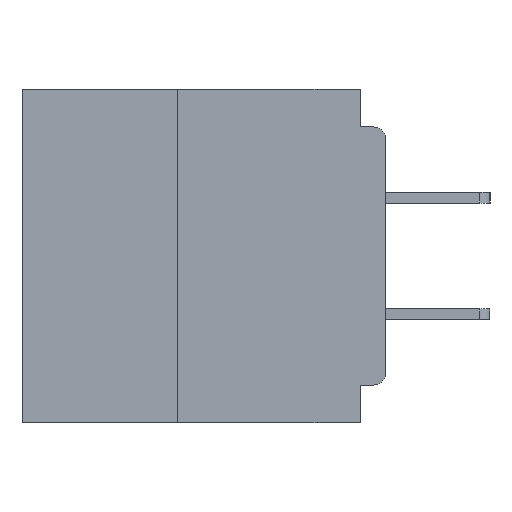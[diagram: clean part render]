
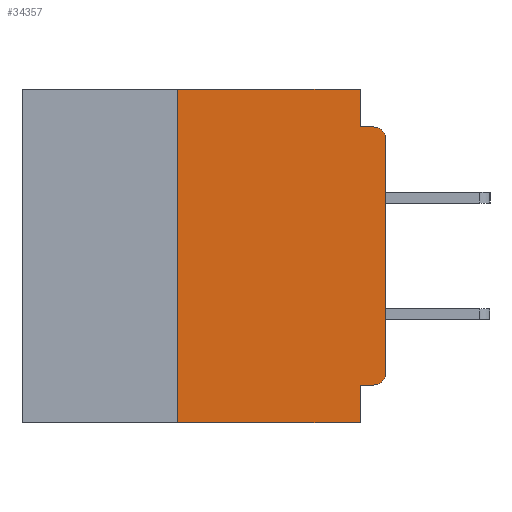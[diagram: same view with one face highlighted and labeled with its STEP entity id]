
A CAD part, left-side view. The second image highlights one B-rep face of the part: STEP entity #34357.
In plain terms, the highlighted planar face has unit normal (-1, 0, 0).
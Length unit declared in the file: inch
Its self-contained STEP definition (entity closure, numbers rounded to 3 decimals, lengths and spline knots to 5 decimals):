
#876 = AXIS2_PLACEMENT_3D ( 'NONE', #6348, #29457, #9717 ) ;
#1422 = DIRECTION ( 'NONE',  ( 1., 0., 0. ) ) ;
#1645 = CARTESIAN_POINT ( 'NONE',  ( 0., 0., -0.06 ) ) ;
#1681 = ORIENTED_EDGE ( 'NONE', *, *, #37611, .T. ) ;
#2135 = VECTOR ( 'NONE', #24964, 39.37008 ) ;
#2602 = LINE ( 'NONE', #12589, #36642 ) ;
#2660 = CARTESIAN_POINT ( 'NONE',  ( 0., 0.25, 0. ) ) ;
#3828 = EDGE_LOOP ( 'NONE', ( #1681, #27173, #12456, #31280, #8950, #22543, #33242, #8551, #8902, #25449 ) ) ;
#4200 = DIRECTION ( 'NONE',  ( 0., 0., -1. ) ) ;
#5131 = CARTESIAN_POINT ( 'NONE',  ( 0., 0.031, -0.4 ) ) ;
#6348 = CARTESIAN_POINT ( 'NONE',  ( 0., 0.015, -0.34 ) ) ;
#7102 = VERTEX_POINT ( 'NONE', #30619 ) ;
#7953 = EDGE_CURVE ( 'NONE', #16757, #12683, #25934, .T. ) ;
#8014 = CARTESIAN_POINT ( 'NONE',  ( 0., 0.437, 0. ) ) ;
#8551 = ORIENTED_EDGE ( 'NONE', *, *, #33032, .F. ) ;
#8730 = DIRECTION ( 'NONE',  ( -1., 0., 0. ) ) ;
#8902 = ORIENTED_EDGE ( 'NONE', *, *, #31078, .F. ) ;
#8950 = ORIENTED_EDGE ( 'NONE', *, *, #7953, .F. ) ;
#9042 = LINE ( 'NONE', #31678, #41821 ) ;
#9165 = FACE_OUTER_BOUND ( 'NONE', #3828, .T. ) ;
#9479 = EDGE_CURVE ( 'NONE', #12995, #27220, #18649, .T. ) ;
#9717 = DIRECTION ( 'NONE',  ( 0., 0., -1. ) ) ;
#9945 = VERTEX_POINT ( 'NONE', #10991 ) ;
#10199 = CIRCLE ( 'NONE', #24313, 0.015 ) ;
#10349 = VECTOR ( 'NONE', #4200, 39.37008 ) ;
#10695 = EDGE_CURVE ( 'NONE', #18546, #7102, #10199, .T. ) ;
#10877 = VECTOR ( 'NONE', #39828, 39.37008 ) ;
#10991 = CARTESIAN_POINT ( 'NONE',  ( 0., 0.25, -0.4 ) ) ;
#11383 = CARTESIAN_POINT ( 'NONE',  ( 0., 0., -0.34 ) ) ;
#11424 = CARTESIAN_POINT ( 'NONE',  ( 0., 0.031, 0. ) ) ;
#12456 = ORIENTED_EDGE ( 'NONE', *, *, #35690, .F. ) ;
#12589 = CARTESIAN_POINT ( 'NONE',  ( 0., 0., -0.355 ) ) ;
#12683 = VERTEX_POINT ( 'NONE', #11424 ) ;
#12995 = VERTEX_POINT ( 'NONE', #32770 ) ;
#15411 = CARTESIAN_POINT ( 'NONE',  ( 0., 0.437, 0. ) ) ;
#16291 = EDGE_CURVE ( 'NONE', #9945, #24626, #19732, .T. ) ;
#16563 = VERTEX_POINT ( 'NONE', #28183 ) ;
#16757 = VERTEX_POINT ( 'NONE', #2660 ) ;
#18546 = VERTEX_POINT ( 'NONE', #1645 ) ;
#18649 = CIRCLE ( 'NONE', #876, 0.015 ) ;
#19203 = LINE ( 'NONE', #30465, #10349 ) ;
#19732 = LINE ( 'NONE', #39680, #10877 ) ;
#20570 = CARTESIAN_POINT ( 'NONE',  ( 0., 0.031, -0.045 ) ) ;
#22029 = DIRECTION ( 'NONE',  ( 0., -1., 0. ) ) ;
#22543 = ORIENTED_EDGE ( 'NONE', *, *, #23143, .F. ) ;
#22972 = LINE ( 'NONE', #37022, #39219 ) ;
#23143 = EDGE_CURVE ( 'NONE', #9945, #16757, #22972, .T. ) ;
#24313 = AXIS2_PLACEMENT_3D ( 'NONE', #28531, #8730, #31767 ) ;
#24428 = VERTEX_POINT ( 'NONE', #20570 ) ;
#24626 = VERTEX_POINT ( 'NONE', #5131 ) ;
#24662 = DIRECTION ( 'NONE',  ( 0., 0., -1. ) ) ;
#24964 = DIRECTION ( 'NONE',  ( 0., 0., -1. ) ) ;
#25087 = VECTOR ( 'NONE', #36261, 39.37008 ) ;
#25449 = ORIENTED_EDGE ( 'NONE', *, *, #9479, .T. ) ;
#25934 = LINE ( 'NONE', #15411, #42156 ) ;
#27173 = ORIENTED_EDGE ( 'NONE', *, *, #10695, .T. ) ;
#27220 = VERTEX_POINT ( 'NONE', #11383 ) ;
#28183 = CARTESIAN_POINT ( 'NONE',  ( 0., 0.031, -0.355 ) ) ;
#28531 = CARTESIAN_POINT ( 'NONE',  ( 0., 0.015, -0.06 ) ) ;
#28980 = DIRECTION ( 'NONE',  ( 0., 1., 0. ) ) ;
#29457 = DIRECTION ( 'NONE',  ( -1., 0., 0. ) ) ;
#30465 = CARTESIAN_POINT ( 'NONE',  ( 0., 0.031, -0.4 ) ) ;
#30619 = CARTESIAN_POINT ( 'NONE',  ( 0., 0.015, -0.045 ) ) ;
#31046 = AXIS2_PLACEMENT_3D ( 'NONE', #8014, #1422, #24662 ) ;
#31078 = EDGE_CURVE ( 'NONE', #12995, #16563, #2602, .T. ) ;
#31280 = ORIENTED_EDGE ( 'NONE', *, *, #38584, .F. ) ;
#31678 = CARTESIAN_POINT ( 'NONE',  ( 0., 0., -0.045 ) ) ;
#31767 = DIRECTION ( 'NONE',  ( 0., 0., -1. ) ) ;
#32770 = CARTESIAN_POINT ( 'NONE',  ( 0., 0.015, -0.355 ) ) ;
#32991 = CARTESIAN_POINT ( 'NONE',  ( 0., 0., 0. ) ) ;
#33032 = EDGE_CURVE ( 'NONE', #16563, #24626, #19203, .T. ) ;
#33242 = ORIENTED_EDGE ( 'NONE', *, *, #16291, .T. ) ;
#34357 = ADVANCED_FACE ( 'NONE', ( #9165 ), #40840, .F. ) ;
#34736 = LINE ( 'NONE', #32991, #25087 ) ;
#34931 = DIRECTION ( 'NONE',  ( 0., -1., 0. ) ) ;
#35690 = EDGE_CURVE ( 'NONE', #24428, #7102, #9042, .T. ) ;
#36261 = DIRECTION ( 'NONE',  ( 0., 0., 1. ) ) ;
#36642 = VECTOR ( 'NONE', #28980, 39.37008 ) ;
#37022 = CARTESIAN_POINT ( 'NONE',  ( 0., 0.25, -0.4 ) ) ;
#37208 = LINE ( 'NONE', #37910, #2135 ) ;
#37611 = EDGE_CURVE ( 'NONE', #27220, #18546, #34736, .T. ) ;
#37910 = CARTESIAN_POINT ( 'NONE',  ( 0., 0.031, 0. ) ) ;
#38584 = EDGE_CURVE ( 'NONE', #12683, #24428, #37208, .T. ) ;
#39219 = VECTOR ( 'NONE', #40271, 39.37008 ) ;
#39680 = CARTESIAN_POINT ( 'NONE',  ( 0., 0.437, -0.4 ) ) ;
#39828 = DIRECTION ( 'NONE',  ( 0., -1., 0. ) ) ;
#40271 = DIRECTION ( 'NONE',  ( 0., 0., 1. ) ) ;
#40840 = PLANE ( 'NONE',  #31046 ) ;
#41821 = VECTOR ( 'NONE', #34931, 39.37008 ) ;
#42156 = VECTOR ( 'NONE', #22029, 39.37008 ) ;
